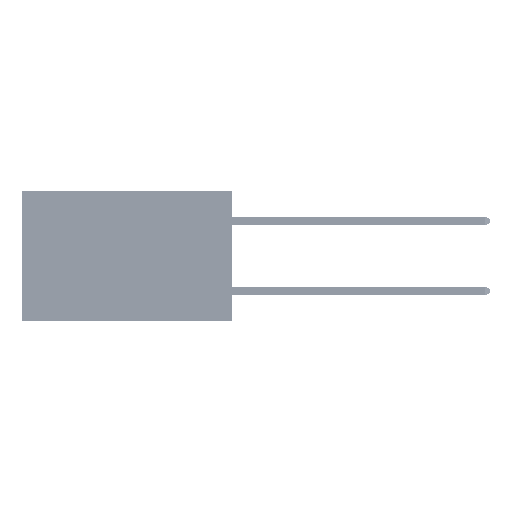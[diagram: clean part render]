
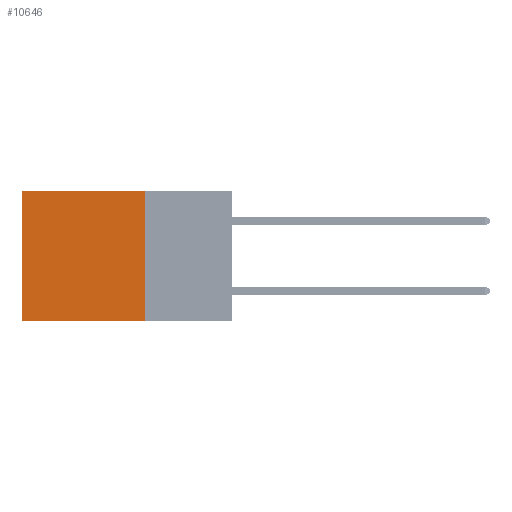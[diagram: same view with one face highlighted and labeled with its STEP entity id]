
A CAD part, left-side view. The second image highlights one B-rep face of the part: STEP entity #10646.
In plain terms, the highlighted planar face has unit normal (-1, 0, 0).
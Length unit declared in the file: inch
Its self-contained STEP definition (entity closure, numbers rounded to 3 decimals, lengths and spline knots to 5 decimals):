
#722 = DIRECTION ( 'NONE',  ( 0., 0., -1. ) ) ;
#1406 = ORIENTED_EDGE ( 'NONE', *, *, #38530, .T. ) ;
#1578 = EDGE_CURVE ( 'NONE', #37388, #44267, #16275, .T. ) ;
#2895 = CARTESIAN_POINT ( 'NONE',  ( 0.2875, 0.6, -0.37 ) ) ;
#8590 = CARTESIAN_POINT ( 'NONE',  ( 0.2875, 0.25, 0. ) ) ;
#10646 = ADVANCED_FACE ( 'NONE', ( #41070 ), #37355, .F. ) ;
#11063 = VECTOR ( 'NONE', #722, 39.37008 ) ;
#14541 = DIRECTION ( 'NONE',  ( 0., 1., 0. ) ) ;
#15255 = CARTESIAN_POINT ( 'NONE',  ( 0.2875, 0.25, 0. ) ) ;
#16275 = LINE ( 'NONE', #8590, #11063 ) ;
#16653 = EDGE_CURVE ( 'NONE', #37388, #48442, #37971, .T. ) ;
#18696 = CARTESIAN_POINT ( 'NONE',  ( 0.2875, 0.25, 0. ) ) ;
#20354 = VECTOR ( 'NONE', #37113, 39.37008 ) ;
#22094 = LINE ( 'NONE', #25983, #20354 ) ;
#22276 = AXIS2_PLACEMENT_3D ( 'NONE', #18696, #41278, #22475 ) ;
#22475 = DIRECTION ( 'NONE',  ( 0., 0., -1. ) ) ;
#23723 = ORIENTED_EDGE ( 'NONE', *, *, #1578, .F. ) ;
#24037 = EDGE_LOOP ( 'NONE', ( #1406, #31710, #23723, #35379 ) ) ;
#25983 = CARTESIAN_POINT ( 'NONE',  ( 0.2875, 0.25, -0.37 ) ) ;
#26863 = VECTOR ( 'NONE', #31180, 39.37008 ) ;
#28564 = VECTOR ( 'NONE', #14541, 39.37008 ) ;
#31180 = DIRECTION ( 'NONE',  ( 0., 0., -1. ) ) ;
#31710 = ORIENTED_EDGE ( 'NONE', *, *, #39389, .F. ) ;
#33378 = VERTEX_POINT ( 'NONE', #2895 ) ;
#35379 = ORIENTED_EDGE ( 'NONE', *, *, #16653, .T. ) ;
#35784 = CARTESIAN_POINT ( 'NONE',  ( 0.2875, 0.25, -0.37 ) ) ;
#36273 = LINE ( 'NONE', #46845, #26863 ) ;
#37113 = DIRECTION ( 'NONE',  ( 0., 1., 0. ) ) ;
#37355 = PLANE ( 'NONE',  #22276 ) ;
#37388 = VERTEX_POINT ( 'NONE', #15255 ) ;
#37971 = LINE ( 'NONE', #44512, #28564 ) ;
#38530 = EDGE_CURVE ( 'NONE', #48442, #33378, #36273, .T. ) ;
#39389 = EDGE_CURVE ( 'NONE', #44267, #33378, #22094, .T. ) ;
#41070 = FACE_OUTER_BOUND ( 'NONE', #24037, .T. ) ;
#41278 = DIRECTION ( 'NONE',  ( 1., 0., 0. ) ) ;
#43819 = CARTESIAN_POINT ( 'NONE',  ( 0.2875, 0.6, 0. ) ) ;
#44267 = VERTEX_POINT ( 'NONE', #35784 ) ;
#44512 = CARTESIAN_POINT ( 'NONE',  ( 0.2875, 0.25, 0. ) ) ;
#46845 = CARTESIAN_POINT ( 'NONE',  ( 0.2875, 0.6, 0. ) ) ;
#48442 = VERTEX_POINT ( 'NONE', #43819 ) ;
